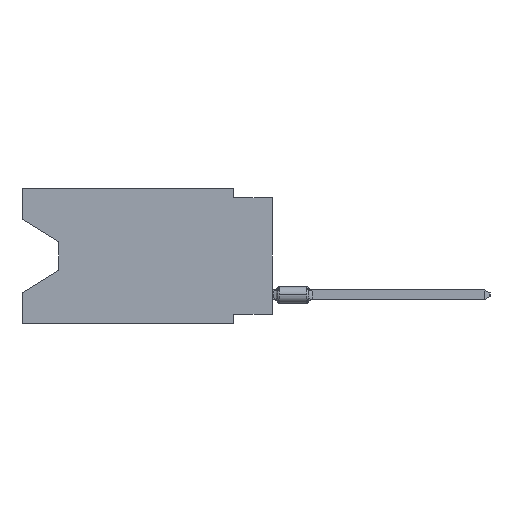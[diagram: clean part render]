
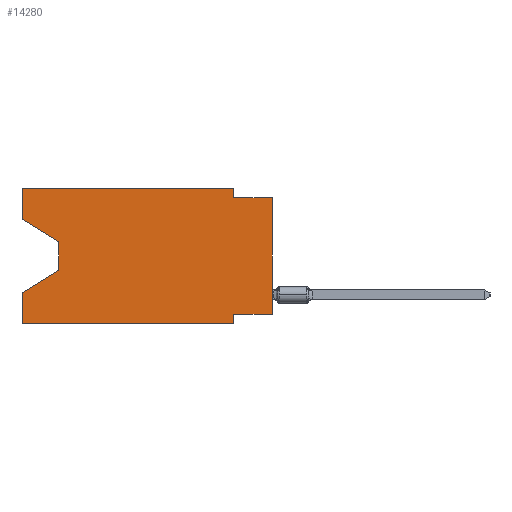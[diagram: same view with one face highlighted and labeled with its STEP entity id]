
A CAD part, left-side view. The second image highlights one B-rep face of the part: STEP entity #14280.
In plain terms, the highlighted planar face has unit normal (-1, 0, 0).
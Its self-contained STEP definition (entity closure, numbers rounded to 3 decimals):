
#716 = EDGE_CURVE ( 'NONE', #38993, #3448, #6026, .T. ) ;
#1526 = CARTESIAN_POINT ( 'NONE',  ( 0., 16.383, -2.038 ) ) ;
#2018 = VECTOR ( 'NONE', #39402, 1000. ) ;
#3448 = VERTEX_POINT ( 'NONE', #17847 ) ;
#3748 = CARTESIAN_POINT ( 'NONE',  ( 0., 16.383, 0. ) ) ;
#4311 = EDGE_CURVE ( 'NONE', #37324, #10481, #7703, .T. ) ;
#5300 = LINE ( 'NONE', #17611, #21734 ) ;
#6026 = LINE ( 'NONE', #18751, #21385 ) ;
#7174 = EDGE_CURVE ( 'NONE', #30058, #10481, #13319, .T. ) ;
#7318 = ORIENTED_EDGE ( 'NONE', *, *, #17968, .T. ) ;
#7397 = EDGE_CURVE ( 'NONE', #26150, #9027, #33346, .T. ) ;
#7703 = LINE ( 'NONE', #33803, #19571 ) ;
#8012 = LINE ( 'NONE', #1526, #32987 ) ;
#8082 = CARTESIAN_POINT ( 'NONE',  ( 0., 13.97, -5.385 ) ) ;
#9027 = VERTEX_POINT ( 'NONE', #27035 ) ;
#9133 = CARTESIAN_POINT ( 'NONE',  ( 0., 16.383, -8.89 ) ) ;
#9659 = CARTESIAN_POINT ( 'NONE',  ( 0., 13.97, -3.505 ) ) ;
#9709 = ORIENTED_EDGE ( 'NONE', *, *, #27191, .F. ) ;
#9756 = VECTOR ( 'NONE', #35696, 1000. ) ;
#10451 = PLANE ( 'NONE',  #13270 ) ;
#10481 = VERTEX_POINT ( 'NONE', #39631 ) ;
#11368 = EDGE_LOOP ( 'NONE', ( #29878, #7318, #41224, #21271, #41353, #14253, #18713, #27209, #30209, #12508, #22584, #9709 ) ) ;
#12427 = VERTEX_POINT ( 'NONE', #9659 ) ;
#12508 = ORIENTED_EDGE ( 'NONE', *, *, #37870, .F. ) ;
#12908 = CARTESIAN_POINT ( 'NONE',  ( 0., 0., -0.635 ) ) ;
#13270 = AXIS2_PLACEMENT_3D ( 'NONE', #39078, #30263, #39683 ) ;
#13319 = LINE ( 'NONE', #12908, #30348 ) ;
#13454 = CARTESIAN_POINT ( 'NONE',  ( 0., 16.383, -2.038 ) ) ;
#14193 = CARTESIAN_POINT ( 'NONE',  ( 0., 16.383, -8.89 ) ) ;
#14253 = ORIENTED_EDGE ( 'NONE', *, *, #22517, .F. ) ;
#14280 = ADVANCED_FACE ( 'NONE', ( #39281 ), #10451, .F. ) ;
#14416 = VECTOR ( 'NONE', #33764, 1000. ) ;
#15365 = DIRECTION ( 'NONE',  ( 0., 0., -1. ) ) ;
#15570 = LINE ( 'NONE', #25198, #19552 ) ;
#16392 = VECTOR ( 'NONE', #33409, 1000. ) ;
#16772 = CARTESIAN_POINT ( 'NONE',  ( 0., 2.54, -8.255 ) ) ;
#17286 = DIRECTION ( 'NONE',  ( 0., 0., 1. ) ) ;
#17611 = CARTESIAN_POINT ( 'NONE',  ( 0., 2.54, 0. ) ) ;
#17847 = CARTESIAN_POINT ( 'NONE',  ( 0., 2.54, 0. ) ) ;
#17968 = EDGE_CURVE ( 'NONE', #12427, #26150, #26467, .T. ) ;
#18028 = DIRECTION ( 'NONE',  ( 0., 0., 1. ) ) ;
#18226 = CARTESIAN_POINT ( 'NONE',  ( 0., 0., -8.255 ) ) ;
#18490 = CARTESIAN_POINT ( 'NONE',  ( 0., 16.383, 0. ) ) ;
#18713 = ORIENTED_EDGE ( 'NONE', *, *, #32016, .F. ) ;
#18751 = CARTESIAN_POINT ( 'NONE',  ( 0., 16.383, 0. ) ) ;
#19552 = VECTOR ( 'NONE', #15365, 1000. ) ;
#19571 = VECTOR ( 'NONE', #17286, 1000. ) ;
#20528 = DIRECTION ( 'NONE',  ( 0., -0.855, -0.519 ) ) ;
#20970 = VERTEX_POINT ( 'NONE', #16772 ) ;
#21166 = DIRECTION ( 'NONE',  ( 0., 0., -1. ) ) ;
#21271 = ORIENTED_EDGE ( 'NONE', *, *, #31471, .F. ) ;
#21385 = VECTOR ( 'NONE', #41335, 1000. ) ;
#21734 = VECTOR ( 'NONE', #21166, 1000. ) ;
#21797 = CARTESIAN_POINT ( 'NONE',  ( 0., 16.383, 0. ) ) ;
#22517 = EDGE_CURVE ( 'NONE', #20970, #37127, #15570, .T. ) ;
#22584 = ORIENTED_EDGE ( 'NONE', *, *, #716, .F. ) ;
#23301 = CARTESIAN_POINT ( 'NONE',  ( 0., 13.97, -3.505 ) ) ;
#23720 = VECTOR ( 'NONE', #18028, 1000. ) ;
#25198 = CARTESIAN_POINT ( 'NONE',  ( 0., 2.54, -8.89 ) ) ;
#25609 = EDGE_CURVE ( 'NONE', #32253, #37127, #39496, .T. ) ;
#26150 = VERTEX_POINT ( 'NONE', #28318 ) ;
#26286 = DIRECTION ( 'NONE',  ( 0., -1., 0. ) ) ;
#26467 = LINE ( 'NONE', #23301, #2018 ) ;
#27035 = CARTESIAN_POINT ( 'NONE',  ( 0., 16.383, -6.852 ) ) ;
#27191 = EDGE_CURVE ( 'NONE', #40951, #38993, #31449, .T. ) ;
#27209 = ORIENTED_EDGE ( 'NONE', *, *, #4311, .T. ) ;
#27293 = DIRECTION ( 'NONE',  ( 0., 0.855, -0.519 ) ) ;
#28280 = LINE ( 'NONE', #21797, #23720 ) ;
#28318 = CARTESIAN_POINT ( 'NONE',  ( 0., 13.97, -5.385 ) ) ;
#29878 = ORIENTED_EDGE ( 'NONE', *, *, #35855, .T. ) ;
#30058 = VERTEX_POINT ( 'NONE', #32893 ) ;
#30209 = ORIENTED_EDGE ( 'NONE', *, *, #7174, .F. ) ;
#30263 = DIRECTION ( 'NONE',  ( 1., 0., 0. ) ) ;
#30348 = VECTOR ( 'NONE', #26286, 1000. ) ;
#31449 = LINE ( 'NONE', #18490, #14416 ) ;
#31471 = EDGE_CURVE ( 'NONE', #32253, #9027, #28280, .T. ) ;
#32016 = EDGE_CURVE ( 'NONE', #37324, #20970, #36103, .T. ) ;
#32253 = VERTEX_POINT ( 'NONE', #9133 ) ;
#32893 = CARTESIAN_POINT ( 'NONE',  ( 0., 2.54, -0.635 ) ) ;
#32987 = VECTOR ( 'NONE', #20528, 1000. ) ;
#33346 = LINE ( 'NONE', #8082, #35703 ) ;
#33409 = DIRECTION ( 'NONE',  ( 0., -1., 0. ) ) ;
#33764 = DIRECTION ( 'NONE',  ( 0., 0., 1. ) ) ;
#33803 = CARTESIAN_POINT ( 'NONE',  ( 0., 0., 0. ) ) ;
#34908 = CARTESIAN_POINT ( 'NONE',  ( 0., 0., -8.255 ) ) ;
#35696 = DIRECTION ( 'NONE',  ( 0., 1., 0. ) ) ;
#35703 = VECTOR ( 'NONE', #27293, 1000. ) ;
#35855 = EDGE_CURVE ( 'NONE', #40951, #12427, #8012, .T. ) ;
#36103 = LINE ( 'NONE', #34908, #9756 ) ;
#36836 = CARTESIAN_POINT ( 'NONE',  ( 0., 2.54, -8.89 ) ) ;
#37127 = VERTEX_POINT ( 'NONE', #36836 ) ;
#37324 = VERTEX_POINT ( 'NONE', #18226 ) ;
#37870 = EDGE_CURVE ( 'NONE', #3448, #30058, #5300, .T. ) ;
#38993 = VERTEX_POINT ( 'NONE', #3748 ) ;
#39078 = CARTESIAN_POINT ( 'NONE',  ( 0., 16.383, 0. ) ) ;
#39281 = FACE_OUTER_BOUND ( 'NONE', #11368, .T. ) ;
#39402 = DIRECTION ( 'NONE',  ( 0., 0., -1. ) ) ;
#39496 = LINE ( 'NONE', #14193, #16392 ) ;
#39631 = CARTESIAN_POINT ( 'NONE',  ( 0., 0., -0.635 ) ) ;
#39683 = DIRECTION ( 'NONE',  ( 0., 0., -1. ) ) ;
#40951 = VERTEX_POINT ( 'NONE', #13454 ) ;
#41224 = ORIENTED_EDGE ( 'NONE', *, *, #7397, .T. ) ;
#41335 = DIRECTION ( 'NONE',  ( 0., -1., 0. ) ) ;
#41353 = ORIENTED_EDGE ( 'NONE', *, *, #25609, .T. ) ;
